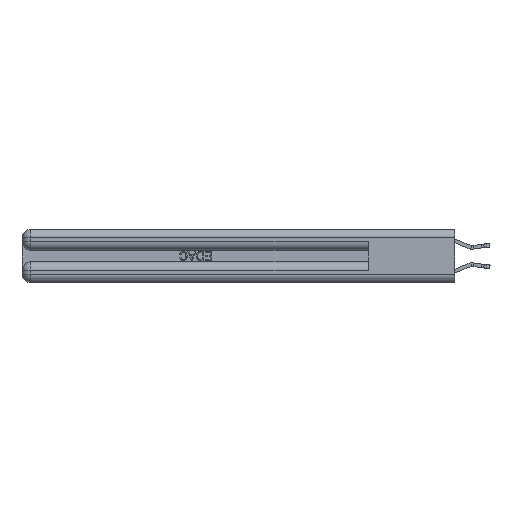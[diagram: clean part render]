
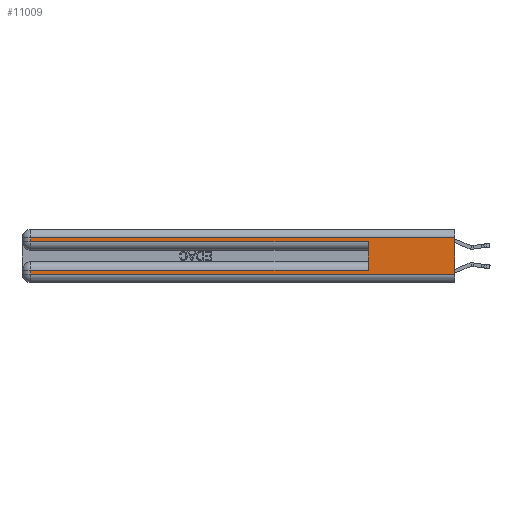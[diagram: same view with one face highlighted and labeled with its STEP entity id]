
A CAD part, left-side view. The second image highlights one B-rep face of the part: STEP entity #11009.
In plain terms, the highlighted planar face has unit normal (-1, 0, 0).
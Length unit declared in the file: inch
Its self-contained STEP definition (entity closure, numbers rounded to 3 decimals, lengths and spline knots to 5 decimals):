
#76 = EDGE_CURVE ( 'NONE', #4861, #15690, #16676, .T. ) ;
#844 = LINE ( 'NONE', #33574, #5824 ) ;
#1716 = CARTESIAN_POINT ( 'NONE',  ( 0., 0., 0.37 ) ) ;
#3102 = DIRECTION ( 'NONE',  ( 0., 0., -1. ) ) ;
#3504 = CARTESIAN_POINT ( 'NONE',  ( 0., 2.94, 0.37 ) ) ;
#4479 = LINE ( 'NONE', #1716, #18812 ) ;
#4861 = VERTEX_POINT ( 'NONE', #31459 ) ;
#4893 = VECTOR ( 'NONE', #10862, 39.37008 ) ;
#5096 = ORIENTED_EDGE ( 'NONE', *, *, #16793, .T. ) ;
#5824 = VECTOR ( 'NONE', #13821, 39.37008 ) ;
#6922 = DIRECTION ( 'NONE',  ( 1., 0., 0. ) ) ;
#7130 = CARTESIAN_POINT ( 'NONE',  ( 0., 0., 0.06 ) ) ;
#7143 = CARTESIAN_POINT ( 'NONE',  ( 0., 0.6, 0.285 ) ) ;
#7152 = CARTESIAN_POINT ( 'NONE',  ( 0., 0., 0.085 ) ) ;
#7943 = ORIENTED_EDGE ( 'NONE', *, *, #33786, .T. ) ;
#8179 = LINE ( 'NONE', #31832, #4893 ) ;
#9454 = PLANE ( 'NONE',  #19530 ) ;
#9579 = DIRECTION ( 'NONE',  ( 0., 0., -1. ) ) ;
#9609 = FACE_OUTER_BOUND ( 'NONE', #32008, .T. ) ;
#9650 = VECTOR ( 'NONE', #3102, 39.37008 ) ;
#9725 = VECTOR ( 'NONE', #13970, 39.37008 ) ;
#10429 = VECTOR ( 'NONE', #14055, 39.37008 ) ;
#10862 = DIRECTION ( 'NONE',  ( 0., -1., 0. ) ) ;
#11009 = ADVANCED_FACE ( 'NONE', ( #9609 ), #9454, .F. ) ;
#11418 = CARTESIAN_POINT ( 'NONE',  ( 0., 0., 0.31 ) ) ;
#12068 = VERTEX_POINT ( 'NONE', #7143 ) ;
#13764 = VERTEX_POINT ( 'NONE', #21505 ) ;
#13821 = DIRECTION ( 'NONE',  ( 0., 0., 1. ) ) ;
#13970 = DIRECTION ( 'NONE',  ( 0., 0., -1. ) ) ;
#14037 = EDGE_CURVE ( 'NONE', #21493, #4861, #31986, .T. ) ;
#14055 = DIRECTION ( 'NONE',  ( 0., 1., 0. ) ) ;
#15683 = ORIENTED_EDGE ( 'NONE', *, *, #27490, .T. ) ;
#15690 = VERTEX_POINT ( 'NONE', #16876 ) ;
#15950 = VERTEX_POINT ( 'NONE', #7130 ) ;
#16676 = LINE ( 'NONE', #3504, #9725 ) ;
#16790 = VECTOR ( 'NONE', #33069, 39.37008 ) ;
#16793 = EDGE_CURVE ( 'NONE', #13764, #17188, #28927, .T. ) ;
#16867 = ORIENTED_EDGE ( 'NONE', *, *, #24887, .F. ) ;
#16876 = CARTESIAN_POINT ( 'NONE',  ( 0., 2.94, 0.06 ) ) ;
#17188 = VERTEX_POINT ( 'NONE', #17898 ) ;
#17304 = ORIENTED_EDGE ( 'NONE', *, *, #28933, .T. ) ;
#17406 = VERTEX_POINT ( 'NONE', #24420 ) ;
#17504 = VECTOR ( 'NONE', #18428, 39.37008 ) ;
#17535 = DIRECTION ( 'NONE',  ( 0., 0., -1. ) ) ;
#17898 = CARTESIAN_POINT ( 'NONE',  ( 0., 2.94, 0.285 ) ) ;
#18428 = DIRECTION ( 'NONE',  ( 0., -1., 0. ) ) ;
#18587 = ORIENTED_EDGE ( 'NONE', *, *, #14037, .T. ) ;
#18812 = VECTOR ( 'NONE', #17535, 39.37008 ) ;
#19530 = AXIS2_PLACEMENT_3D ( 'NONE', #25287, #6922, #9579 ) ;
#20589 = EDGE_CURVE ( 'NONE', #17406, #15950, #4479, .T. ) ;
#21493 = VERTEX_POINT ( 'NONE', #25828 ) ;
#21505 = CARTESIAN_POINT ( 'NONE',  ( 0., 2.94, 0.31 ) ) ;
#24420 = CARTESIAN_POINT ( 'NONE',  ( 0., 0., 0.31 ) ) ;
#24887 = EDGE_CURVE ( 'NONE', #21493, #12068, #844, .T. ) ;
#25287 = CARTESIAN_POINT ( 'NONE',  ( 0., 0., 0.37 ) ) ;
#25290 = ORIENTED_EDGE ( 'NONE', *, *, #76, .T. ) ;
#25828 = CARTESIAN_POINT ( 'NONE',  ( 0., 0.6, 0.085 ) ) ;
#27490 = EDGE_CURVE ( 'NONE', #17188, #12068, #33112, .T. ) ;
#28927 = LINE ( 'NONE', #31797, #9650 ) ;
#28933 = EDGE_CURVE ( 'NONE', #17406, #13764, #33018, .T. ) ;
#29864 = ORIENTED_EDGE ( 'NONE', *, *, #20589, .F. ) ;
#31459 = CARTESIAN_POINT ( 'NONE',  ( 0., 2.94, 0.085 ) ) ;
#31496 = CARTESIAN_POINT ( 'NONE',  ( 0., 0., 0.285 ) ) ;
#31797 = CARTESIAN_POINT ( 'NONE',  ( 0., 2.94, 0.37 ) ) ;
#31832 = CARTESIAN_POINT ( 'NONE',  ( 0., 0., 0.06 ) ) ;
#31986 = LINE ( 'NONE', #7152, #16790 ) ;
#32008 = EDGE_LOOP ( 'NONE', ( #29864, #17304, #5096, #15683, #16867, #18587, #25290, #7943 ) ) ;
#33018 = LINE ( 'NONE', #11418, #10429 ) ;
#33069 = DIRECTION ( 'NONE',  ( 0., 1., 0. ) ) ;
#33112 = LINE ( 'NONE', #31496, #17504 ) ;
#33574 = CARTESIAN_POINT ( 'NONE',  ( 0., 0.6, 0.145 ) ) ;
#33786 = EDGE_CURVE ( 'NONE', #15690, #15950, #8179, .T. ) ;
